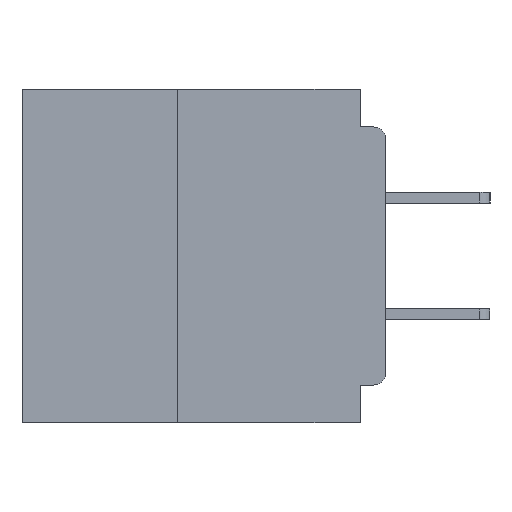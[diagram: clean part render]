
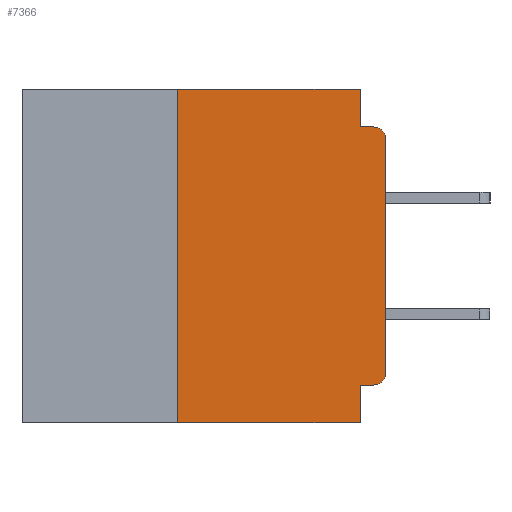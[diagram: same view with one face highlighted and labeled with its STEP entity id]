
A CAD part, left-side view. The second image highlights one B-rep face of the part: STEP entity #7366.
In plain terms, the highlighted planar face has unit normal (-1, 0, 0).
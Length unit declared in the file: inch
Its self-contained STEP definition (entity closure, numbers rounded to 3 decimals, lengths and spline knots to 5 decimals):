
#937 = VERTEX_POINT ( 'NONE', #30587 ) ;
#1046 = AXIS2_PLACEMENT_3D ( 'NONE', #11511, #15101, #39882 ) ;
#1221 = CARTESIAN_POINT ( 'NONE',  ( 0., 0.437, -0.4 ) ) ;
#1317 = VECTOR ( 'NONE', #41503, 39.37008 ) ;
#1639 = ORIENTED_EDGE ( 'NONE', *, *, #38285, .T. ) ;
#2076 = VERTEX_POINT ( 'NONE', #13542 ) ;
#2724 = DIRECTION ( 'NONE',  ( 0., -1., 0. ) ) ;
#3629 = CARTESIAN_POINT ( 'NONE',  ( 0., 0.031, 0. ) ) ;
#4727 = VERTEX_POINT ( 'NONE', #30851 ) ;
#4816 = VERTEX_POINT ( 'NONE', #19232 ) ;
#5589 = DIRECTION ( 'NONE',  ( -1., 0., 0. ) ) ;
#6268 = AXIS2_PLACEMENT_3D ( 'NONE', #26828, #5589, #30408 ) ;
#6504 = VERTEX_POINT ( 'NONE', #34856 ) ;
#6770 = VECTOR ( 'NONE', #36746, 39.37008 ) ;
#7366 = ADVANCED_FACE ( 'NONE', ( #32789 ), #32772, .F. ) ;
#7922 = CARTESIAN_POINT ( 'NONE',  ( 0., 0.015, -0.34 ) ) ;
#9080 = CARTESIAN_POINT ( 'NONE',  ( 0., 0.031, 0. ) ) ;
#10388 = ORIENTED_EDGE ( 'NONE', *, *, #39550, .T. ) ;
#10702 = LINE ( 'NONE', #37937, #1317 ) ;
#11511 = CARTESIAN_POINT ( 'NONE',  ( 0., 0.437, 0. ) ) ;
#11534 = DIRECTION ( 'NONE',  ( 0., 0., -1. ) ) ;
#11956 = CARTESIAN_POINT ( 'NONE',  ( 0., 0.437, 0. ) ) ;
#12499 = LINE ( 'NONE', #44764, #30238 ) ;
#12727 = ORIENTED_EDGE ( 'NONE', *, *, #22358, .F. ) ;
#12786 = DIRECTION ( 'NONE',  ( 0., 1., 0. ) ) ;
#13228 = ORIENTED_EDGE ( 'NONE', *, *, #16658, .F. ) ;
#13436 = CARTESIAN_POINT ( 'NONE',  ( 0., 0., -0.045 ) ) ;
#13542 = CARTESIAN_POINT ( 'NONE',  ( 0., 0.031, -0.355 ) ) ;
#15101 = DIRECTION ( 'NONE',  ( 1., 0., 0. ) ) ;
#15939 = EDGE_CURVE ( 'NONE', #937, #26070, #12499, .T. ) ;
#16018 = CARTESIAN_POINT ( 'NONE',  ( 0., 0.031, -0.4 ) ) ;
#16350 = CARTESIAN_POINT ( 'NONE',  ( 0., 0., -0.355 ) ) ;
#16471 = DIRECTION ( 'NONE',  ( 0., 0., 1. ) ) ;
#16658 = EDGE_CURVE ( 'NONE', #38888, #6504, #10702, .T. ) ;
#17205 = EDGE_LOOP ( 'NONE', ( #45652, #26935, #43000, #30855, #27561, #13228, #10388, #39268, #12727, #1639 ) ) ;
#17921 = EDGE_CURVE ( 'NONE', #26070, #4816, #32314, .T. ) ;
#18628 = LINE ( 'NONE', #13436, #45669 ) ;
#19232 = CARTESIAN_POINT ( 'NONE',  ( 0., 0.015, -0.045 ) ) ;
#22358 = EDGE_CURVE ( 'NONE', #45315, #2076, #45594, .T. ) ;
#22476 = DIRECTION ( 'NONE',  ( 0., -1., 0. ) ) ;
#22849 = EDGE_CURVE ( 'NONE', #6504, #39986, #34007, .T. ) ;
#23397 = DIRECTION ( 'NONE',  ( 0., 0., -1. ) ) ;
#23539 = LINE ( 'NONE', #16018, #42312 ) ;
#24158 = AXIS2_PLACEMENT_3D ( 'NONE', #7922, #32795, #11534 ) ;
#26070 = VERTEX_POINT ( 'NONE', #41932 ) ;
#26828 = CARTESIAN_POINT ( 'NONE',  ( 0., 0.015, -0.06 ) ) ;
#26832 = VECTOR ( 'NONE', #12786, 39.37008 ) ;
#26935 = ORIENTED_EDGE ( 'NONE', *, *, #17921, .T. ) ;
#27561 = ORIENTED_EDGE ( 'NONE', *, *, #22849, .F. ) ;
#28737 = LINE ( 'NONE', #1221, #45309 ) ;
#29282 = VECTOR ( 'NONE', #23397, 39.37008 ) ;
#30238 = VECTOR ( 'NONE', #16471, 39.37008 ) ;
#30408 = DIRECTION ( 'NONE',  ( 0., 0., -1. ) ) ;
#30587 = CARTESIAN_POINT ( 'NONE',  ( 0., 0., -0.34 ) ) ;
#30747 = EDGE_CURVE ( 'NONE', #2076, #4727, #23539, .T. ) ;
#30851 = CARTESIAN_POINT ( 'NONE',  ( 0., 0.031, -0.4 ) ) ;
#30855 = ORIENTED_EDGE ( 'NONE', *, *, #39701, .F. ) ;
#32314 = CIRCLE ( 'NONE', #6268, 0.015 ) ;
#32772 = PLANE ( 'NONE',  #1046 ) ;
#32789 = FACE_OUTER_BOUND ( 'NONE', #17205, .T. ) ;
#32795 = DIRECTION ( 'NONE',  ( -1., 0., 0. ) ) ;
#33252 = CIRCLE ( 'NONE', #24158, 0.015 ) ;
#33833 = DIRECTION ( 'NONE',  ( 0., 0., -1. ) ) ;
#34007 = LINE ( 'NONE', #11956, #6770 ) ;
#34855 = EDGE_CURVE ( 'NONE', #44052, #4816, #18628, .T. ) ;
#34856 = CARTESIAN_POINT ( 'NONE',  ( 0., 0.25, 0. ) ) ;
#36465 = CARTESIAN_POINT ( 'NONE',  ( 0., 0.25, -0.4 ) ) ;
#36746 = DIRECTION ( 'NONE',  ( 0., -1., 0. ) ) ;
#37236 = CARTESIAN_POINT ( 'NONE',  ( 0., 0.031, -0.045 ) ) ;
#37937 = CARTESIAN_POINT ( 'NONE',  ( 0., 0.25, -0.4 ) ) ;
#38285 = EDGE_CURVE ( 'NONE', #45315, #937, #33252, .T. ) ;
#38695 = LINE ( 'NONE', #9080, #29282 ) ;
#38888 = VERTEX_POINT ( 'NONE', #36465 ) ;
#39268 = ORIENTED_EDGE ( 'NONE', *, *, #30747, .F. ) ;
#39550 = EDGE_CURVE ( 'NONE', #38888, #4727, #28737, .T. ) ;
#39701 = EDGE_CURVE ( 'NONE', #39986, #44052, #38695, .T. ) ;
#39882 = DIRECTION ( 'NONE',  ( 0., 0., -1. ) ) ;
#39986 = VERTEX_POINT ( 'NONE', #3629 ) ;
#41320 = CARTESIAN_POINT ( 'NONE',  ( 0., 0.015, -0.355 ) ) ;
#41503 = DIRECTION ( 'NONE',  ( 0., 0., 1. ) ) ;
#41932 = CARTESIAN_POINT ( 'NONE',  ( 0., 0., -0.06 ) ) ;
#42312 = VECTOR ( 'NONE', #33833, 39.37008 ) ;
#43000 = ORIENTED_EDGE ( 'NONE', *, *, #34855, .F. ) ;
#44052 = VERTEX_POINT ( 'NONE', #37236 ) ;
#44764 = CARTESIAN_POINT ( 'NONE',  ( 0., 0., 0. ) ) ;
#45309 = VECTOR ( 'NONE', #22476, 39.37008 ) ;
#45315 = VERTEX_POINT ( 'NONE', #41320 ) ;
#45594 = LINE ( 'NONE', #16350, #26832 ) ;
#45652 = ORIENTED_EDGE ( 'NONE', *, *, #15939, .T. ) ;
#45669 = VECTOR ( 'NONE', #2724, 39.37008 ) ;
